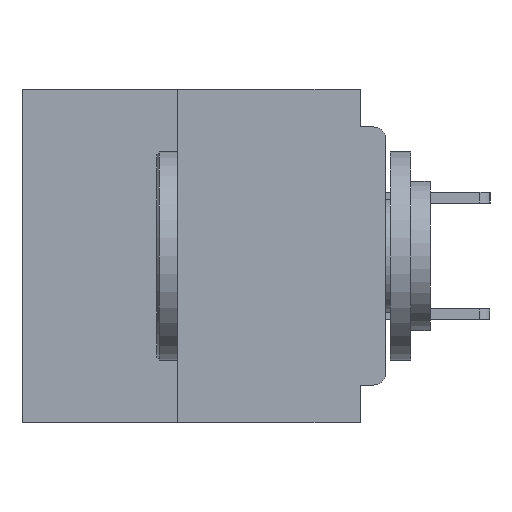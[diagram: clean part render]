
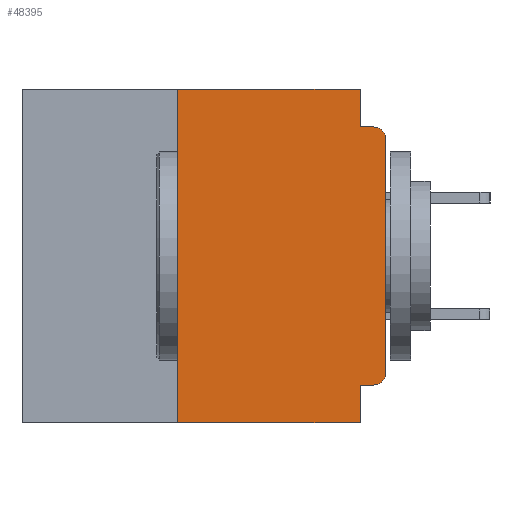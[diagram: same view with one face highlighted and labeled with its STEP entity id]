
A CAD part, left-side view. The second image highlights one B-rep face of the part: STEP entity #48395.
In plain terms, the highlighted planar face has unit normal (-1, 0, 0).
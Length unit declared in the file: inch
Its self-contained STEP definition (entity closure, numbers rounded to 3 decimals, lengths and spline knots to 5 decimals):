
#299 = VECTOR ( 'NONE', #38746, 39.37008 ) ;
#606 = CARTESIAN_POINT ( 'NONE',  ( 0., 0.031, 0. ) ) ;
#1318 = CARTESIAN_POINT ( 'NONE',  ( 0., 0.25, 0. ) ) ;
#1369 = EDGE_CURVE ( 'NONE', #9527, #22627, #23301, .T. ) ;
#2080 = VERTEX_POINT ( 'NONE', #41463 ) ;
#2906 = CARTESIAN_POINT ( 'NONE',  ( 0., 0.25, -0.4 ) ) ;
#3609 = DIRECTION ( 'NONE',  ( -1., 0., 0. ) ) ;
#3821 = CARTESIAN_POINT ( 'NONE',  ( 0., 0., -0.34 ) ) ;
#4508 = EDGE_CURVE ( 'NONE', #21583, #12876, #7642, .T. ) ;
#4823 = PLANE ( 'NONE',  #12067 ) ;
#5042 = DIRECTION ( 'NONE',  ( 0., 0., -1. ) ) ;
#6276 = CARTESIAN_POINT ( 'NONE',  ( 0., 0.015, -0.355 ) ) ;
#7123 = DIRECTION ( 'NONE',  ( 0., 1., 0. ) ) ;
#7481 = CARTESIAN_POINT ( 'NONE',  ( 0., 0., -0.06 ) ) ;
#7642 = LINE ( 'NONE', #7844, #18111 ) ;
#7844 = CARTESIAN_POINT ( 'NONE',  ( 0., 0., 0. ) ) ;
#9034 = LINE ( 'NONE', #21837, #54714 ) ;
#9298 = DIRECTION ( 'NONE',  ( 0., 0., -1. ) ) ;
#9527 = VERTEX_POINT ( 'NONE', #51732 ) ;
#11184 = ORIENTED_EDGE ( 'NONE', *, *, #39117, .F. ) ;
#11353 = CARTESIAN_POINT ( 'NONE',  ( 0., 0.031, -0.4 ) ) ;
#11972 = CARTESIAN_POINT ( 'NONE',  ( 0., 0.437, -0.4 ) ) ;
#12067 = AXIS2_PLACEMENT_3D ( 'NONE', #22569, #35903, #9298 ) ;
#12073 = LINE ( 'NONE', #11972, #299 ) ;
#12165 = DIRECTION ( 'NONE',  ( 0., 0., -1. ) ) ;
#12660 = VERTEX_POINT ( 'NONE', #44920 ) ;
#12876 = VERTEX_POINT ( 'NONE', #7481 ) ;
#13105 = AXIS2_PLACEMENT_3D ( 'NONE', #30238, #3609, #34658 ) ;
#13406 = CARTESIAN_POINT ( 'NONE',  ( 0., 0.437, 0. ) ) ;
#14127 = EDGE_CURVE ( 'NONE', #35181, #39867, #46451, .T. ) ;
#15512 = VECTOR ( 'NONE', #5042, 39.37008 ) ;
#16131 = ORIENTED_EDGE ( 'NONE', *, *, #51586, .T. ) ;
#16864 = ORIENTED_EDGE ( 'NONE', *, *, #4508, .T. ) ;
#17042 = DIRECTION ( 'NONE',  ( -1., 0., 0. ) ) ;
#17896 = DIRECTION ( 'NONE',  ( 0., -1., 0. ) ) ;
#18111 = VECTOR ( 'NONE', #56553, 39.37008 ) ;
#19178 = EDGE_CURVE ( 'NONE', #39867, #2080, #27239, .T. ) ;
#20393 = CARTESIAN_POINT ( 'NONE',  ( 0., 0., -0.355 ) ) ;
#20458 = CARTESIAN_POINT ( 'NONE',  ( 0., 0.031, -0.4 ) ) ;
#20845 = AXIS2_PLACEMENT_3D ( 'NONE', #43565, #17042, #48003 ) ;
#21583 = VERTEX_POINT ( 'NONE', #3821 ) ;
#21837 = CARTESIAN_POINT ( 'NONE',  ( 0., 0., -0.045 ) ) ;
#22569 = CARTESIAN_POINT ( 'NONE',  ( 0., 0.437, 0. ) ) ;
#22627 = VERTEX_POINT ( 'NONE', #20458 ) ;
#22815 = VECTOR ( 'NONE', #7123, 39.37008 ) ;
#23132 = ORIENTED_EDGE ( 'NONE', *, *, #1369, .F. ) ;
#23301 = LINE ( 'NONE', #11353, #33705 ) ;
#24522 = ORIENTED_EDGE ( 'NONE', *, *, #48722, .F. ) ;
#24741 = VERTEX_POINT ( 'NONE', #36162 ) ;
#25835 = EDGE_CURVE ( 'NONE', #12876, #12660, #34442, .T. ) ;
#27184 = EDGE_CURVE ( 'NONE', #2080, #24741, #27365, .T. ) ;
#27239 = LINE ( 'NONE', #13406, #49306 ) ;
#27365 = LINE ( 'NONE', #606, #15512 ) ;
#27721 = FACE_OUTER_BOUND ( 'NONE', #42288, .T. ) ;
#28660 = ORIENTED_EDGE ( 'NONE', *, *, #19178, .F. ) ;
#30238 = CARTESIAN_POINT ( 'NONE',  ( 0., 0.015, -0.34 ) ) ;
#33705 = VECTOR ( 'NONE', #12165, 39.37008 ) ;
#34442 = CIRCLE ( 'NONE', #20845, 0.015 ) ;
#34658 = DIRECTION ( 'NONE',  ( 0., 0., -1. ) ) ;
#35169 = DIRECTION ( 'NONE',  ( 0., -1., 0. ) ) ;
#35181 = VERTEX_POINT ( 'NONE', #36129 ) ;
#35903 = DIRECTION ( 'NONE',  ( 1., 0., 0. ) ) ;
#36129 = CARTESIAN_POINT ( 'NONE',  ( 0., 0.25, -0.4 ) ) ;
#36162 = CARTESIAN_POINT ( 'NONE',  ( 0., 0.031, -0.045 ) ) ;
#38746 = DIRECTION ( 'NONE',  ( 0., -1., 0. ) ) ;
#39117 = EDGE_CURVE ( 'NONE', #24741, #12660, #9034, .T. ) ;
#39867 = VERTEX_POINT ( 'NONE', #1318 ) ;
#41463 = CARTESIAN_POINT ( 'NONE',  ( 0., 0.031, 0. ) ) ;
#42288 = EDGE_LOOP ( 'NONE', ( #16864, #44591, #11184, #50711, #28660, #45883, #16131, #23132, #24522, #53531 ) ) ;
#43565 = CARTESIAN_POINT ( 'NONE',  ( 0., 0.015, -0.06 ) ) ;
#44591 = ORIENTED_EDGE ( 'NONE', *, *, #25835, .T. ) ;
#44920 = CARTESIAN_POINT ( 'NONE',  ( 0., 0.015, -0.045 ) ) ;
#45883 = ORIENTED_EDGE ( 'NONE', *, *, #14127, .F. ) ;
#46451 = LINE ( 'NONE', #2906, #56726 ) ;
#48003 = DIRECTION ( 'NONE',  ( 0., 0., -1. ) ) ;
#48191 = CIRCLE ( 'NONE', #13105, 0.015 ) ;
#48395 = ADVANCED_FACE ( 'NONE', ( #27721 ), #4823, .F. ) ;
#48722 = EDGE_CURVE ( 'NONE', #57211, #9527, #56584, .T. ) ;
#49306 = VECTOR ( 'NONE', #17896, 39.37008 ) ;
#50711 = ORIENTED_EDGE ( 'NONE', *, *, #27184, .F. ) ;
#51586 = EDGE_CURVE ( 'NONE', #35181, #22627, #12073, .T. ) ;
#51732 = CARTESIAN_POINT ( 'NONE',  ( 0., 0.031, -0.355 ) ) ;
#53531 = ORIENTED_EDGE ( 'NONE', *, *, #55345, .T. ) ;
#54714 = VECTOR ( 'NONE', #35169, 39.37008 ) ;
#55345 = EDGE_CURVE ( 'NONE', #57211, #21583, #48191, .T. ) ;
#55898 = DIRECTION ( 'NONE',  ( 0., 0., 1. ) ) ;
#56553 = DIRECTION ( 'NONE',  ( 0., 0., 1. ) ) ;
#56584 = LINE ( 'NONE', #20393, #22815 ) ;
#56726 = VECTOR ( 'NONE', #55898, 39.37008 ) ;
#57211 = VERTEX_POINT ( 'NONE', #6276 ) ;
